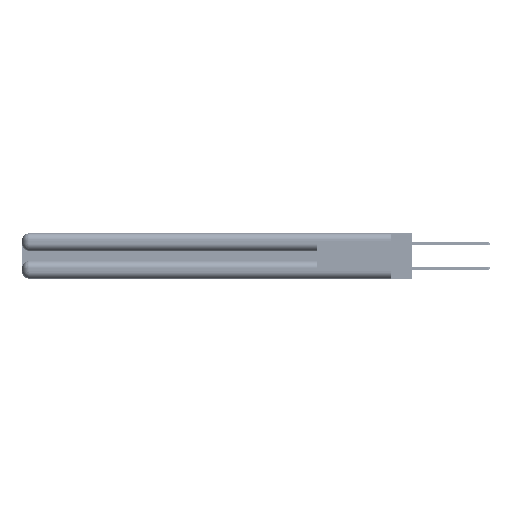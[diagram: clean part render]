
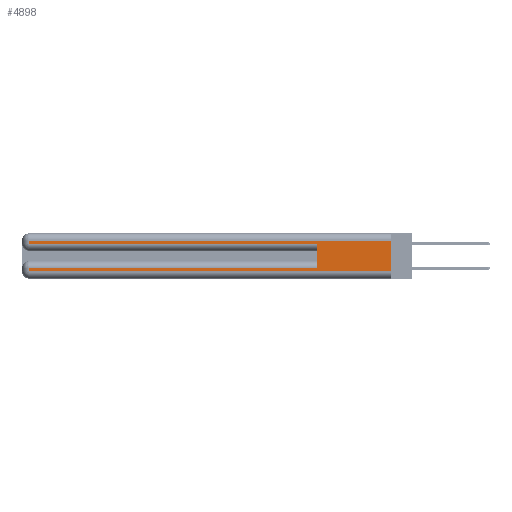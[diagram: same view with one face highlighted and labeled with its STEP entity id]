
A CAD part, left-side view. The second image highlights one B-rep face of the part: STEP entity #4898.
In plain terms, the highlighted planar face has unit normal (-1, 0, 0).
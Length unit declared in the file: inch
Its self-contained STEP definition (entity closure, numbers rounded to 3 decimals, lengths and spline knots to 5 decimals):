
#285 = CARTESIAN_POINT ( 'NONE',  ( 0., 0., 0.31 ) ) ;
#313 = EDGE_CURVE ( 'NONE', #31724, #33320, #50283, .T. ) ;
#858 = VERTEX_POINT ( 'NONE', #285 ) ;
#2248 = CARTESIAN_POINT ( 'NONE',  ( 0., 2.94, 0.37 ) ) ;
#2987 = CARTESIAN_POINT ( 'NONE',  ( 0., 0., 0.285 ) ) ;
#4898 = ADVANCED_FACE ( 'NONE', ( #46659 ), #33660, .F. ) ;
#5134 = CARTESIAN_POINT ( 'NONE',  ( 0., 0., 0.06 ) ) ;
#8573 = DIRECTION ( 'NONE',  ( 0., 0., -1. ) ) ;
#8586 = CARTESIAN_POINT ( 'NONE',  ( 0., 0., 0.085 ) ) ;
#8869 = LINE ( 'NONE', #20914, #17831 ) ;
#9547 = VECTOR ( 'NONE', #30830, 39.37008 ) ;
#10263 = LINE ( 'NONE', #13352, #24209 ) ;
#11501 = VECTOR ( 'NONE', #34517, 39.37008 ) ;
#11916 = VECTOR ( 'NONE', #36963, 39.37008 ) ;
#12646 = EDGE_CURVE ( 'NONE', #50987, #45452, #24641, .T. ) ;
#13340 = VERTEX_POINT ( 'NONE', #23759 ) ;
#13352 = CARTESIAN_POINT ( 'NONE',  ( 0., 2.94, 0.37 ) ) ;
#13400 = CARTESIAN_POINT ( 'NONE',  ( 0., 2.94, 0.31 ) ) ;
#13858 = EDGE_LOOP ( 'NONE', ( #25561, #17967, #42178, #18597, #20809, #30595, #33830, #15808 ) ) ;
#14540 = DIRECTION ( 'NONE',  ( 0., 1., 0. ) ) ;
#14635 = LINE ( 'NONE', #26395, #43873 ) ;
#15808 = ORIENTED_EDGE ( 'NONE', *, *, #313, .T. ) ;
#17831 = VECTOR ( 'NONE', #21268, 39.37008 ) ;
#17907 = DIRECTION ( 'NONE',  ( 0., 0., 1. ) ) ;
#17967 = ORIENTED_EDGE ( 'NONE', *, *, #19136, .T. ) ;
#18597 = ORIENTED_EDGE ( 'NONE', *, *, #20001, .T. ) ;
#19136 = EDGE_CURVE ( 'NONE', #858, #50554, #14635, .T. ) ;
#20001 = EDGE_CURVE ( 'NONE', #35570, #45452, #29158, .T. ) ;
#20809 = ORIENTED_EDGE ( 'NONE', *, *, #12646, .F. ) ;
#20914 = CARTESIAN_POINT ( 'NONE',  ( 0., 0., 0.37 ) ) ;
#21268 = DIRECTION ( 'NONE',  ( 0., 0., -1. ) ) ;
#21462 = CARTESIAN_POINT ( 'NONE',  ( 0., 0., 0.37 ) ) ;
#23759 = CARTESIAN_POINT ( 'NONE',  ( 0., 2.94, 0.085 ) ) ;
#24209 = VECTOR ( 'NONE', #8573, 39.37008 ) ;
#24220 = AXIS2_PLACEMENT_3D ( 'NONE', #21462, #37585, #30812 ) ;
#24641 = LINE ( 'NONE', #29066, #27190 ) ;
#25561 = ORIENTED_EDGE ( 'NONE', *, *, #35797, .F. ) ;
#25854 = CARTESIAN_POINT ( 'NONE',  ( 0., 0., 0.06 ) ) ;
#26382 = CARTESIAN_POINT ( 'NONE',  ( 0., 0.6, 0.285 ) ) ;
#26395 = CARTESIAN_POINT ( 'NONE',  ( 0., 0., 0.31 ) ) ;
#27190 = VECTOR ( 'NONE', #17907, 39.37008 ) ;
#27830 = LINE ( 'NONE', #8586, #11916 ) ;
#29066 = CARTESIAN_POINT ( 'NONE',  ( 0., 0.6, 0.145 ) ) ;
#29158 = LINE ( 'NONE', #2987, #34813 ) ;
#29962 = EDGE_CURVE ( 'NONE', #50987, #13340, #27830, .T. ) ;
#30595 = ORIENTED_EDGE ( 'NONE', *, *, #29962, .T. ) ;
#30812 = DIRECTION ( 'NONE',  ( 0., 0., -1. ) ) ;
#30830 = DIRECTION ( 'NONE',  ( 0., 0., -1. ) ) ;
#31724 = VERTEX_POINT ( 'NONE', #32615 ) ;
#32615 = CARTESIAN_POINT ( 'NONE',  ( 0., 2.94, 0.06 ) ) ;
#33320 = VERTEX_POINT ( 'NONE', #5134 ) ;
#33660 = PLANE ( 'NONE',  #24220 ) ;
#33830 = ORIENTED_EDGE ( 'NONE', *, *, #35663, .T. ) ;
#34517 = DIRECTION ( 'NONE',  ( 0., -1., 0. ) ) ;
#34813 = VECTOR ( 'NONE', #35272, 39.37008 ) ;
#35272 = DIRECTION ( 'NONE',  ( 0., -1., 0. ) ) ;
#35570 = VERTEX_POINT ( 'NONE', #39182 ) ;
#35663 = EDGE_CURVE ( 'NONE', #13340, #31724, #48901, .T. ) ;
#35797 = EDGE_CURVE ( 'NONE', #858, #33320, #8869, .T. ) ;
#36963 = DIRECTION ( 'NONE',  ( 0., 1., 0. ) ) ;
#37585 = DIRECTION ( 'NONE',  ( 1., 0., 0. ) ) ;
#39182 = CARTESIAN_POINT ( 'NONE',  ( 0., 2.94, 0.285 ) ) ;
#41287 = EDGE_CURVE ( 'NONE', #50554, #35570, #10263, .T. ) ;
#42178 = ORIENTED_EDGE ( 'NONE', *, *, #41287, .T. ) ;
#43873 = VECTOR ( 'NONE', #14540, 39.37008 ) ;
#45452 = VERTEX_POINT ( 'NONE', #26382 ) ;
#46659 = FACE_OUTER_BOUND ( 'NONE', #13858, .T. ) ;
#48901 = LINE ( 'NONE', #2248, #9547 ) ;
#50283 = LINE ( 'NONE', #25854, #11501 ) ;
#50554 = VERTEX_POINT ( 'NONE', #13400 ) ;
#50987 = VERTEX_POINT ( 'NONE', #52219 ) ;
#52219 = CARTESIAN_POINT ( 'NONE',  ( 0., 0.6, 0.085 ) ) ;
